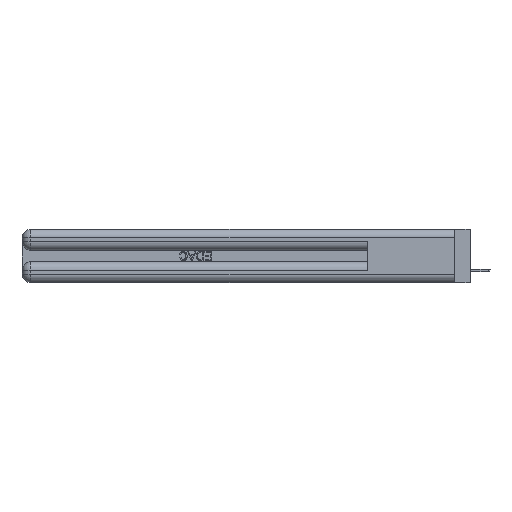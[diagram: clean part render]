
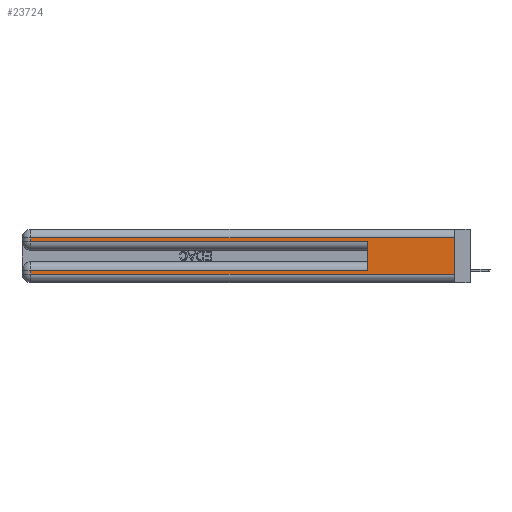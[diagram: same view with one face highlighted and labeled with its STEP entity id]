
A CAD part, left-side view. The second image highlights one B-rep face of the part: STEP entity #23724.
In plain terms, the highlighted planar face has unit normal (-1, 0, 0).
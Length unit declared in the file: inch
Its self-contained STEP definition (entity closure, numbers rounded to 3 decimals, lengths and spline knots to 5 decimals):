
#158 = CARTESIAN_POINT ( 'NONE',  ( 0., 0., 0.285 ) ) ;
#482 = EDGE_CURVE ( 'NONE', #38623, #7482, #28489, .T. ) ;
#1603 = VECTOR ( 'NONE', #31715, 39.37008 ) ;
#2639 = DIRECTION ( 'NONE',  ( 0., 0., -1. ) ) ;
#2662 = VECTOR ( 'NONE', #30115, 39.37008 ) ;
#3784 = LINE ( 'NONE', #158, #16512 ) ;
#4655 = EDGE_CURVE ( 'NONE', #7583, #7482, #27673, .T. ) ;
#5631 = CARTESIAN_POINT ( 'NONE',  ( 0., 2.94, 0.285 ) ) ;
#7373 = CARTESIAN_POINT ( 'NONE',  ( 0., 0., 0.06 ) ) ;
#7482 = VERTEX_POINT ( 'NONE', #8048 ) ;
#7583 = VERTEX_POINT ( 'NONE', #30528 ) ;
#7819 = ORIENTED_EDGE ( 'NONE', *, *, #482, .T. ) ;
#7970 = EDGE_CURVE ( 'NONE', #7583, #38609, #32720, .T. ) ;
#8048 = CARTESIAN_POINT ( 'NONE',  ( 0., 0., 0.06 ) ) ;
#8179 = EDGE_LOOP ( 'NONE', ( #42007, #37381, #42762, #33904, #19348, #11403, #28133, #7819 ) ) ;
#11353 = VECTOR ( 'NONE', #23426, 39.37008 ) ;
#11403 = ORIENTED_EDGE ( 'NONE', *, *, #50372, .T. ) ;
#11615 = CARTESIAN_POINT ( 'NONE',  ( 0., 0., 0.31 ) ) ;
#12914 = LINE ( 'NONE', #54865, #2662 ) ;
#15600 = CARTESIAN_POINT ( 'NONE',  ( 0., 2.94, 0.37 ) ) ;
#16512 = VECTOR ( 'NONE', #24646, 39.37008 ) ;
#16857 = AXIS2_PLACEMENT_3D ( 'NONE', #44232, #27020, #48662 ) ;
#19348 = ORIENTED_EDGE ( 'NONE', *, *, #46178, .F. ) ;
#19627 = CARTESIAN_POINT ( 'NONE',  ( 0., 0., 0.37 ) ) ;
#21541 = VECTOR ( 'NONE', #36305, 39.37008 ) ;
#22490 = EDGE_CURVE ( 'NONE', #38609, #47879, #53093, .T. ) ;
#23426 = DIRECTION ( 'NONE',  ( 0., 1., 0. ) ) ;
#23724 = ADVANCED_FACE ( 'NONE', ( #26467 ), #52563, .F. ) ;
#24646 = DIRECTION ( 'NONE',  ( 0., -1., 0. ) ) ;
#24679 = DIRECTION ( 'NONE',  ( 0., 1., 0. ) ) ;
#25208 = CARTESIAN_POINT ( 'NONE',  ( 0., 2.94, 0.085 ) ) ;
#25440 = VERTEX_POINT ( 'NONE', #35563 ) ;
#26467 = FACE_OUTER_BOUND ( 'NONE', #8179, .T. ) ;
#27020 = DIRECTION ( 'NONE',  ( 1., 0., 0. ) ) ;
#27673 = LINE ( 'NONE', #19627, #31258 ) ;
#28133 = ORIENTED_EDGE ( 'NONE', *, *, #29328, .T. ) ;
#28489 = LINE ( 'NONE', #7373, #38563 ) ;
#29328 = EDGE_CURVE ( 'NONE', #52801, #38623, #45747, .T. ) ;
#30115 = DIRECTION ( 'NONE',  ( 0., 0., 1. ) ) ;
#30528 = CARTESIAN_POINT ( 'NONE',  ( 0., 0., 0.31 ) ) ;
#31258 = VECTOR ( 'NONE', #2639, 39.37008 ) ;
#31715 = DIRECTION ( 'NONE',  ( 0., 0., -1. ) ) ;
#31742 = LINE ( 'NONE', #35357, #11353 ) ;
#32720 = LINE ( 'NONE', #11615, #49607 ) ;
#33904 = ORIENTED_EDGE ( 'NONE', *, *, #48425, .T. ) ;
#35357 = CARTESIAN_POINT ( 'NONE',  ( 0., 0., 0.085 ) ) ;
#35563 = CARTESIAN_POINT ( 'NONE',  ( 0., 0.6, 0.085 ) ) ;
#36305 = DIRECTION ( 'NONE',  ( 0., 0., -1. ) ) ;
#37141 = CARTESIAN_POINT ( 'NONE',  ( 0., 2.94, 0.37 ) ) ;
#37381 = ORIENTED_EDGE ( 'NONE', *, *, #7970, .T. ) ;
#38563 = VECTOR ( 'NONE', #49880, 39.37008 ) ;
#38609 = VERTEX_POINT ( 'NONE', #53559 ) ;
#38623 = VERTEX_POINT ( 'NONE', #54114 ) ;
#42007 = ORIENTED_EDGE ( 'NONE', *, *, #4655, .F. ) ;
#42762 = ORIENTED_EDGE ( 'NONE', *, *, #22490, .T. ) ;
#44232 = CARTESIAN_POINT ( 'NONE',  ( 0., 0., 0.37 ) ) ;
#44887 = VERTEX_POINT ( 'NONE', #46521 ) ;
#45747 = LINE ( 'NONE', #37141, #21541 ) ;
#46178 = EDGE_CURVE ( 'NONE', #25440, #44887, #12914, .T. ) ;
#46521 = CARTESIAN_POINT ( 'NONE',  ( 0., 0.6, 0.285 ) ) ;
#47879 = VERTEX_POINT ( 'NONE', #5631 ) ;
#48425 = EDGE_CURVE ( 'NONE', #47879, #44887, #3784, .T. ) ;
#48662 = DIRECTION ( 'NONE',  ( 0., 0., -1. ) ) ;
#49607 = VECTOR ( 'NONE', #24679, 39.37008 ) ;
#49880 = DIRECTION ( 'NONE',  ( 0., -1., 0. ) ) ;
#50372 = EDGE_CURVE ( 'NONE', #25440, #52801, #31742, .T. ) ;
#52563 = PLANE ( 'NONE',  #16857 ) ;
#52801 = VERTEX_POINT ( 'NONE', #25208 ) ;
#53093 = LINE ( 'NONE', #15600, #1603 ) ;
#53559 = CARTESIAN_POINT ( 'NONE',  ( 0., 2.94, 0.31 ) ) ;
#54114 = CARTESIAN_POINT ( 'NONE',  ( 0., 2.94, 0.06 ) ) ;
#54865 = CARTESIAN_POINT ( 'NONE',  ( 0., 0.6, 0.145 ) ) ;
